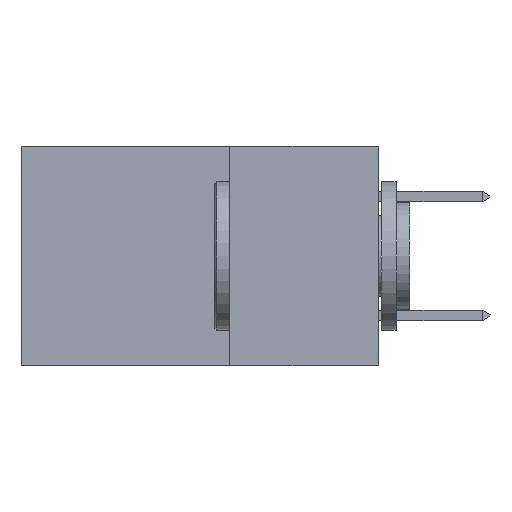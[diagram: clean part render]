
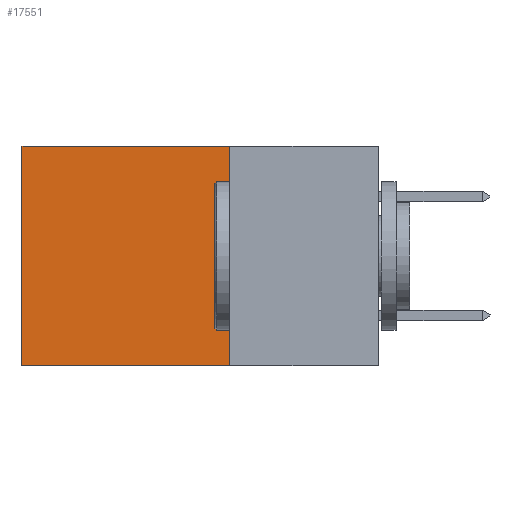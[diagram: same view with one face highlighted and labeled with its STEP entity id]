
A CAD part, left-side view. The second image highlights one B-rep face of the part: STEP entity #17551.
In plain terms, the highlighted planar face has unit normal (-1, 0, 0).
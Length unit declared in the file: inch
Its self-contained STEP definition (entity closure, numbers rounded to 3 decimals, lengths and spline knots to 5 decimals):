
#1585 = LINE ( 'NONE', #23593, #31972 ) ;
#2875 = VERTEX_POINT ( 'NONE', #29699 ) ;
#3602 = CARTESIAN_POINT ( 'NONE',  ( 0.298, 0.25, 0. ) ) ;
#6819 = EDGE_CURVE ( 'NONE', #11694, #9399, #30721, .T. ) ;
#7083 = EDGE_CURVE ( 'NONE', #9399, #8896, #1585, .T. ) ;
#8896 = VERTEX_POINT ( 'NONE', #20887 ) ;
#9399 = VERTEX_POINT ( 'NONE', #18687 ) ;
#9961 = CARTESIAN_POINT ( 'NONE',  ( 0.298, 0.25, 0. ) ) ;
#11694 = VERTEX_POINT ( 'NONE', #9961 ) ;
#11767 = DIRECTION ( 'NONE',  ( 1., 0., 0. ) ) ;
#11866 = ORIENTED_EDGE ( 'NONE', *, *, #18812, .F. ) ;
#12040 = FACE_OUTER_BOUND ( 'NONE', #25055, .T. ) ;
#12547 = CARTESIAN_POINT ( 'NONE',  ( 0.298, 0.25, 0. ) ) ;
#15491 = ORIENTED_EDGE ( 'NONE', *, *, #7083, .T. ) ;
#15656 = DIRECTION ( 'NONE',  ( 0., 0., -1. ) ) ;
#16394 = VECTOR ( 'NONE', #33553, 39.37008 ) ;
#17519 = DIRECTION ( 'NONE',  ( 0., 0., -1. ) ) ;
#17551 = ADVANCED_FACE ( 'NONE', ( #12040 ), #19961, .F. ) ;
#18687 = CARTESIAN_POINT ( 'NONE',  ( 0.298, 0.6, 0. ) ) ;
#18812 = EDGE_CURVE ( 'NONE', #11694, #2875, #21037, .T. ) ;
#19070 = ORIENTED_EDGE ( 'NONE', *, *, #6819, .T. ) ;
#19217 = EDGE_CURVE ( 'NONE', #2875, #8896, #27961, .T. ) ;
#19961 = PLANE ( 'NONE',  #24858 ) ;
#20456 = CARTESIAN_POINT ( 'NONE',  ( 0.298, 0.25, -0.37 ) ) ;
#20887 = CARTESIAN_POINT ( 'NONE',  ( 0.298, 0.6, -0.37 ) ) ;
#21037 = LINE ( 'NONE', #3602, #28794 ) ;
#23593 = CARTESIAN_POINT ( 'NONE',  ( 0.298, 0.6, 0. ) ) ;
#24858 = AXIS2_PLACEMENT_3D ( 'NONE', #32873, #11767, #17519 ) ;
#25055 = EDGE_LOOP ( 'NONE', ( #15491, #27070, #11866, #19070 ) ) ;
#25161 = DIRECTION ( 'NONE',  ( 0., 0., -1. ) ) ;
#25580 = DIRECTION ( 'NONE',  ( 0., 1., 0. ) ) ;
#27070 = ORIENTED_EDGE ( 'NONE', *, *, #19217, .F. ) ;
#27926 = VECTOR ( 'NONE', #25580, 39.37008 ) ;
#27961 = LINE ( 'NONE', #20456, #27926 ) ;
#28794 = VECTOR ( 'NONE', #25161, 39.37008 ) ;
#29699 = CARTESIAN_POINT ( 'NONE',  ( 0.298, 0.25, -0.37 ) ) ;
#30721 = LINE ( 'NONE', #12547, #16394 ) ;
#31972 = VECTOR ( 'NONE', #15656, 39.37008 ) ;
#32873 = CARTESIAN_POINT ( 'NONE',  ( 0.298, 0.25, 0. ) ) ;
#33553 = DIRECTION ( 'NONE',  ( 0., 1., 0. ) ) ;
